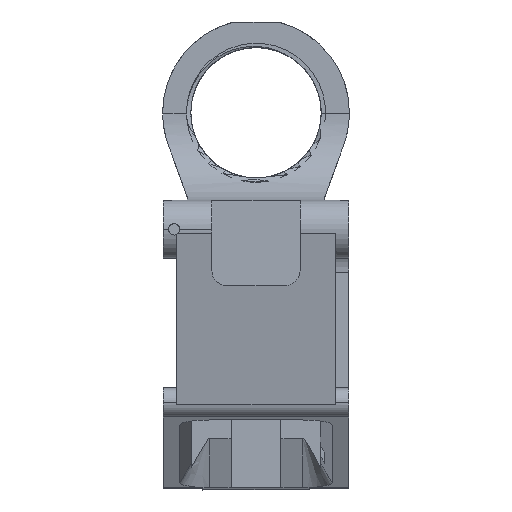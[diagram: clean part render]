
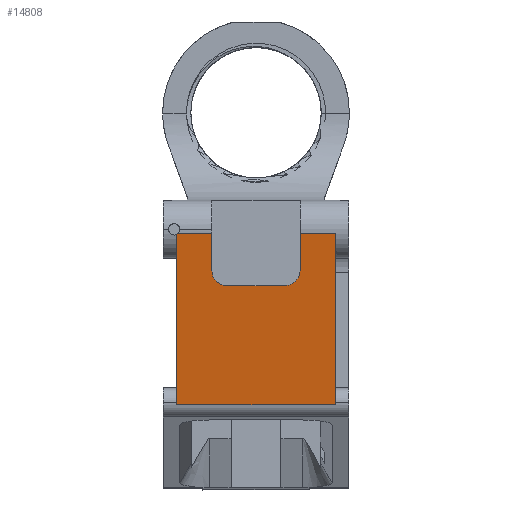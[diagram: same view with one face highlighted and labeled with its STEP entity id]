
A CAD part, top view. The second image highlights one B-rep face of the part: STEP entity #14808.
In plain terms, the highlighted planar face has unit normal (0, -0.156, 0.988).
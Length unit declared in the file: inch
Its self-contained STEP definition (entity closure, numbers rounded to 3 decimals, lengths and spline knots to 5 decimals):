
#373 = EDGE_CURVE ( 'NONE', #16527, #4723, #6177, .T. ) ;
#749 = EDGE_CURVE ( 'NONE', #11782, #5653, #19985, .T. ) ;
#825 = VECTOR ( 'NONE', #16018, 39.37008 ) ;
#830 = ORIENTED_EDGE ( 'NONE', *, *, #7449, .F. ) ;
#870 = VECTOR ( 'NONE', #6297, 39.37008 ) ;
#1020 = DIRECTION ( 'NONE',  ( -1., 0., 0. ) ) ;
#1827 = VECTOR ( 'NONE', #1020, 39.37008 ) ;
#1857 = VERTEX_POINT ( 'NONE', #15142 ) ;
#2441 = EDGE_CURVE ( 'NONE', #8241, #11782, #11140, .T. ) ;
#2513 = ORIENTED_EDGE ( 'NONE', *, *, #10399, .F. ) ;
#2559 = CARTESIAN_POINT ( 'NONE',  ( 0.251, -0.73, 8.89709 ) ) ;
#2581 = CARTESIAN_POINT ( 'NONE',  ( 0.675, -0.28911, 8.96692 ) ) ;
#2873 = ORIENTED_EDGE ( 'NONE', *, *, #19341, .T. ) ;
#2986 = CARTESIAN_POINT ( 'NONE',  ( -0.251, -0.73, 8.89709 ) ) ;
#3233 = CARTESIAN_POINT ( 'NONE',  ( -0.376, -0.28911, 8.96692 ) ) ;
#3336 = FACE_OUTER_BOUND ( 'NONE', #18669, .T. ) ;
#3549 = EDGE_CURVE ( 'NONE', #10712, #6104, #5250, .T. ) ;
#3654 = CARTESIAN_POINT ( 'NONE',  ( 0.32422, -0.73, 8.89709 ) ) ;
#4102 = CARTESIAN_POINT ( 'NONE',  ( 0., -1.74799, 8.73586 ) ) ;
#4336 = VECTOR ( 'NONE', #15862, 39.37008 ) ;
#4723 = VERTEX_POINT ( 'NONE', #19447 ) ;
#5250 = LINE ( 'NONE', #17721, #870 ) ;
#5386 = ORIENTED_EDGE ( 'NONE', *, *, #11350, .T. ) ;
#5433 = VERTEX_POINT ( 'NONE', #5856 ) ;
#5653 = VERTEX_POINT ( 'NONE', #17714 ) ;
#5856 = CARTESIAN_POINT ( 'NONE',  ( 0.376, -0.605, 8.91689 ) ) ;
#6104 = VERTEX_POINT ( 'NONE', #2581 ) ;
#6177 = LINE ( 'NONE', #10811, #1827 ) ;
#6201 = CARTESIAN_POINT ( 'NONE',  ( -0.32422, -0.73, 8.89709 ) ) ;
#6228 = CARTESIAN_POINT ( 'NONE',  ( 0.376, -0.605, 8.91689 ) ) ;
#6275 = CARTESIAN_POINT ( 'NONE',  ( -0.376, -0.67822, 8.90529 ) ) ;
#6277 = VECTOR ( 'NONE', #17158, 39.37008 ) ;
#6297 = DIRECTION ( 'NONE',  ( 0., 0.988, 0.156 ) ) ;
#6319 = PLANE ( 'NONE',  #12074 ) ;
#6434 = CARTESIAN_POINT ( 'NONE',  ( -0.67032, -0.28911, 8.96692 ) ) ;
#6588 =( BOUNDED_CURVE ( )  B_SPLINE_CURVE ( 3, ( #6434, #16228, #21135, #11377 ),
 .UNSPECIFIED., .F., .F. ) 
 B_SPLINE_CURVE_WITH_KNOTS ( ( 4, 4 ),
 ( 5.65037, 5.76554 ),
 .UNSPECIFIED. ) 
 CURVE ( )  GEOMETRIC_REPRESENTATION_ITEM ( )  RATIONAL_B_SPLINE_CURVE ( ( 1., 0.999, 0.999, 1. ) ) 
 REPRESENTATION_ITEM ( '' )  );
#6722 = ORIENTED_EDGE ( 'NONE', *, *, #19938, .T. ) ;
#7449 = EDGE_CURVE ( 'NONE', #5433, #1857, #13375, .T. ) ;
#7528 = ORIENTED_EDGE ( 'NONE', *, *, #17219, .T. ) ;
#7571 = CARTESIAN_POINT ( 'NONE',  ( -0.675, -1.74799, 8.73586 ) ) ;
#7737 = CARTESIAN_POINT ( 'NONE',  ( 0.58425, -0.28911, 8.96692 ) ) ;
#8023 = DIRECTION ( 'NONE',  ( 0., 0.988, 0.156 ) ) ;
#8241 = VERTEX_POINT ( 'NONE', #12019 ) ;
#9214 = ORIENTED_EDGE ( 'NONE', *, *, #10564, .T. ) ;
#9224 = DIRECTION ( 'NONE',  ( 0., 0.988, 0.156 ) ) ;
#9616 = DIRECTION ( 'NONE',  ( 0., -0.156, 0.988 ) ) ;
#10143 = VECTOR ( 'NONE', #9224, 39.37008 ) ;
#10162 = CARTESIAN_POINT ( 'NONE',  ( 0.376, -0.605, 8.91689 ) ) ;
#10176 = ORIENTED_EDGE ( 'NONE', *, *, #373, .T. ) ;
#10399 = EDGE_CURVE ( 'NONE', #12381, #19236, #14460, .T. ) ;
#10468 = ORIENTED_EDGE ( 'NONE', *, *, #2441, .T. ) ;
#10564 = EDGE_CURVE ( 'NONE', #4723, #8241, #14057, .T. ) ;
#10712 = VERTEX_POINT ( 'NONE', #16267 ) ;
#10811 = CARTESIAN_POINT ( 'NONE',  ( 0., -0.73, 8.89709 ) ) ;
#11140 = LINE ( 'NONE', #15988, #18769 ) ;
#11350 = EDGE_CURVE ( 'NONE', #12381, #10712, #14968, .T. ) ;
#11377 = CARTESIAN_POINT ( 'NONE',  ( -0.675, -0.29215, 8.96643 ) ) ;
#11782 = VERTEX_POINT ( 'NONE', #3233 ) ;
#11806 = CARTESIAN_POINT ( 'NONE',  ( 0.376, -0.67822, 8.90529 ) ) ;
#12019 = CARTESIAN_POINT ( 'NONE',  ( -0.376, -0.605, 8.91689 ) ) ;
#12074 = AXIS2_PLACEMENT_3D ( 'NONE', #17746, #9616, #21014 ) ;
#12381 = VERTEX_POINT ( 'NONE', #20166 ) ;
#12911 = CARTESIAN_POINT ( 'NONE',  ( 0., -0.28911, 8.96692 ) ) ;
#13015 = LINE ( 'NONE', #7737, #4336 ) ;
#13375 = LINE ( 'NONE', #6228, #825 ) ;
#13595 = ORIENTED_EDGE ( 'NONE', *, *, #3549, .T. ) ;
#14057 =( BOUNDED_CURVE ( )  B_SPLINE_CURVE ( 3, ( #2986, #6201, #6275, #17699 ),
 .UNSPECIFIED., .F., .F. ) 
 B_SPLINE_CURVE_WITH_KNOTS ( ( 4, 4 ),
 ( 3.14159, 4.71239 ),
 .UNSPECIFIED. ) 
 CURVE ( )  GEOMETRIC_REPRESENTATION_ITEM ( )  RATIONAL_B_SPLINE_CURVE ( ( 1., 0.805, 0.805, 1. ) ) 
 REPRESENTATION_ITEM ( '' )  );
#14079 = CARTESIAN_POINT ( 'NONE',  ( -0.675, -0.29215, 8.96643 ) ) ;
#14460 = LINE ( 'NONE', #7571, #10143 ) ;
#14531 = DIRECTION ( 'NONE',  ( -1., 0., 0. ) ) ;
#14808 = ADVANCED_FACE ( 'NONE', ( #3336 ), #6319, .T. ) ;
#14968 = LINE ( 'NONE', #4102, #6277 ) ;
#15074 = CARTESIAN_POINT ( 'NONE',  ( 0.251, -0.73, 8.89709 ) ) ;
#15142 = CARTESIAN_POINT ( 'NONE',  ( 0.376, -0.28911, 8.96692 ) ) ;
#15329 =( BOUNDED_CURVE ( )  B_SPLINE_CURVE ( 3, ( #10162, #11806, #3654, #15074 ),
 .UNSPECIFIED., .F., .F. ) 
 B_SPLINE_CURVE_WITH_KNOTS ( ( 4, 4 ),
 ( 4.71239, 6.28319 ),
 .UNSPECIFIED. ) 
 CURVE ( )  GEOMETRIC_REPRESENTATION_ITEM ( )  RATIONAL_B_SPLINE_CURVE ( ( 1., 0.805, 0.805, 1. ) ) 
 REPRESENTATION_ITEM ( '' )  );
#15862 = DIRECTION ( 'NONE',  ( -1., 0., 0. ) ) ;
#15988 = CARTESIAN_POINT ( 'NONE',  ( -0.376, -0.28911, 8.96692 ) ) ;
#16018 = DIRECTION ( 'NONE',  ( 0., 0.988, 0.156 ) ) ;
#16228 = CARTESIAN_POINT ( 'NONE',  ( -0.67182, -0.29021, 8.96675 ) ) ;
#16267 = CARTESIAN_POINT ( 'NONE',  ( 0.675, -1.74799, 8.73586 ) ) ;
#16527 = VERTEX_POINT ( 'NONE', #2559 ) ;
#17158 = DIRECTION ( 'NONE',  ( 1., 0., 0. ) ) ;
#17219 = EDGE_CURVE ( 'NONE', #5653, #19236, #6588, .T. ) ;
#17460 = ORIENTED_EDGE ( 'NONE', *, *, #749, .T. ) ;
#17699 = CARTESIAN_POINT ( 'NONE',  ( -0.376, -0.605, 8.91689 ) ) ;
#17714 = CARTESIAN_POINT ( 'NONE',  ( -0.67032, -0.28911, 8.96692 ) ) ;
#17721 = CARTESIAN_POINT ( 'NONE',  ( 0.675, -1.01855, 8.85139 ) ) ;
#17746 = CARTESIAN_POINT ( 'NONE',  ( -0.675, -0.28911, 8.96692 ) ) ;
#18669 = EDGE_LOOP ( 'NONE', ( #9214, #10468, #17460, #7528, #2513, #5386, #13595, #2873, #830, #6722, #10176 ) ) ;
#18769 = VECTOR ( 'NONE', #8023, 39.37008 ) ;
#19236 = VERTEX_POINT ( 'NONE', #14079 ) ;
#19341 = EDGE_CURVE ( 'NONE', #6104, #1857, #13015, .T. ) ;
#19447 = CARTESIAN_POINT ( 'NONE',  ( -0.251, -0.73, 8.89709 ) ) ;
#19459 = VECTOR ( 'NONE', #14531, 39.37008 ) ;
#19938 = EDGE_CURVE ( 'NONE', #5433, #16527, #15329, .T. ) ;
#19985 = LINE ( 'NONE', #12911, #19459 ) ;
#20166 = CARTESIAN_POINT ( 'NONE',  ( -0.675, -1.74799, 8.73586 ) ) ;
#21014 = DIRECTION ( 'NONE',  ( 0., -0.988, -0.156 ) ) ;
#21135 = CARTESIAN_POINT ( 'NONE',  ( -0.67338, -0.29122, 8.96659 ) ) ;
